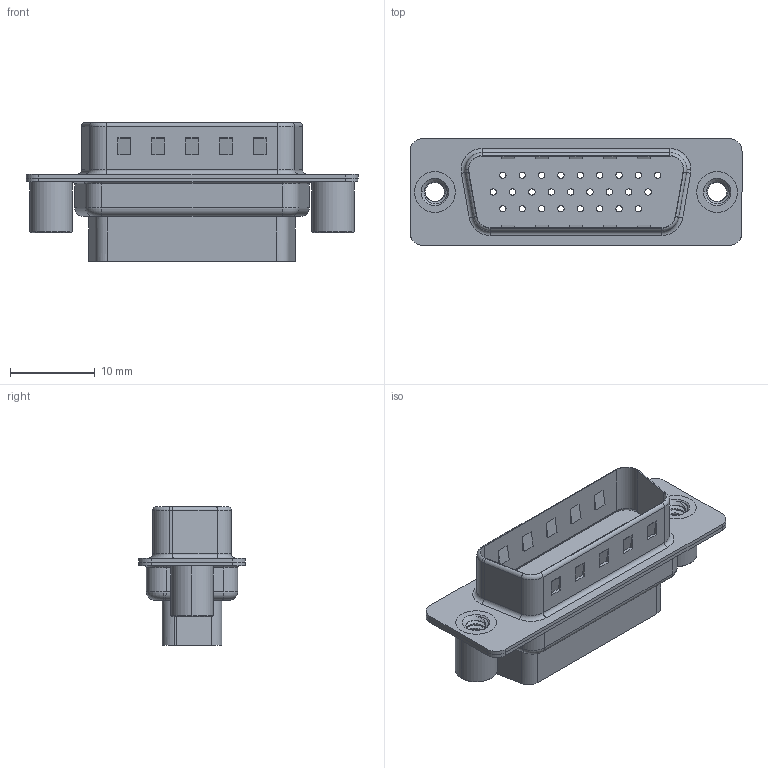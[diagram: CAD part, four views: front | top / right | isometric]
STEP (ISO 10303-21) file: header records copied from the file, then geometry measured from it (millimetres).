
FILE_DESCRIPTION (( 'STEP AP203' ), '1' );
FILE_NAME ('637-026-010-249.STEP', '2020-07-17T21:18:59', ( '' ), ( '' ), 'SwSTEP 2.0', 'SolidWorks 2020', '' );
FILE_SCHEMA (( 'CONFIG_CONTROL_DESIGN' ));
Length unit declared in the file: millimetre
Products named in the file (5): 637 Shell Front_26 Contacts; 637 Housing_26 Contacts HP; 637 4-40 Threaded Standoff BS; 637-026-010-249; 637 Shell Rear_26 Contacts
Assembly tree (5 placements, depth 2):
  637-026-010-249
    637 Housing_26 Contacts HP
    637 Shell Front_26 Contacts
    637 Shell Rear_26 Contacts
    637 4-40 Threaded Standoff BS  x2
Bounding box: 39.2 x 12.6 x 16.4 mm (x, y, z)
Volume: 2146.3 mm3; surface area: 5310.4 mm2
Topology: 5 solids, 5 shells, 570 faces, 1389 edges, 892 vertices
Faces by surface type: cylinder 309, plane 191, torus 50, cone 14, bspline 6
Entity records: 17844 total; most frequent: CARTESIAN_POINT 4419, DIRECTION 2865, ORIENTED_EDGE 2552, EDGE_CURVE 1276, AXIS2_PLACEMENT_3D 1125, VERTEX_POINT 819, EDGE_LOOP 673, VECTOR 615
